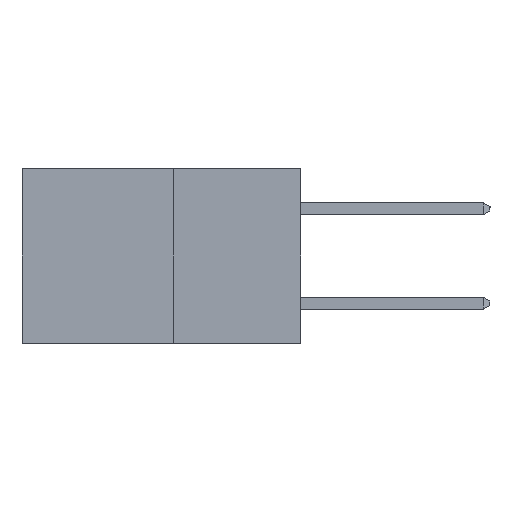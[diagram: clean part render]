
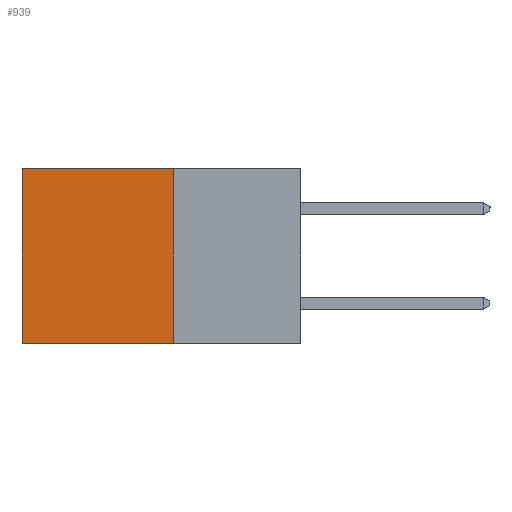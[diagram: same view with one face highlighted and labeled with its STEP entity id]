
A CAD part, left-side view. The second image highlights one B-rep face of the part: STEP entity #939.
In plain terms, the highlighted planar face has unit normal (-1, 0, 0).
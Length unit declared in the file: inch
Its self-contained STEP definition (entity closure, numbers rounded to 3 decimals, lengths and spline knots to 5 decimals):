
#569 = VECTOR ( 'NONE', #7287, 39.37008 ) ;
#777 = CARTESIAN_POINT ( 'NONE',  ( 0.277, 0.27, -0.37 ) ) ;
#939 = ADVANCED_FACE ( 'NONE', ( #9367 ), #11133, .F. ) ;
#1395 = ORIENTED_EDGE ( 'NONE', *, *, #13193, .F. ) ;
#2406 = VERTEX_POINT ( 'NONE', #8641 ) ;
#3998 = VECTOR ( 'NONE', #11134, 39.37008 ) ;
#4005 = VERTEX_POINT ( 'NONE', #13809 ) ;
#4045 = CARTESIAN_POINT ( 'NONE',  ( 0.277, 0.27, -0.37 ) ) ;
#4678 = DIRECTION ( 'NONE',  ( 0., 0., -1. ) ) ;
#5016 = VERTEX_POINT ( 'NONE', #5277 ) ;
#5277 = CARTESIAN_POINT ( 'NONE',  ( 0.277, 0.59, 0. ) ) ;
#5908 = ORIENTED_EDGE ( 'NONE', *, *, #13669, .T. ) ;
#6284 = LINE ( 'NONE', #4045, #6637 ) ;
#6637 = VECTOR ( 'NONE', #13772, 39.37008 ) ;
#7287 = DIRECTION ( 'NONE',  ( 0., 0., -1. ) ) ;
#7516 = AXIS2_PLACEMENT_3D ( 'NONE', #777, #13693, #4678 ) ;
#8641 = CARTESIAN_POINT ( 'NONE',  ( 0.277, 0.27, 0. ) ) ;
#9367 = FACE_OUTER_BOUND ( 'NONE', #10897, .T. ) ;
#9384 = LINE ( 'NONE', #13598, #569 ) ;
#9528 = VECTOR ( 'NONE', #12383, 39.37008 ) ;
#9845 = CARTESIAN_POINT ( 'NONE',  ( 0.277, 0.59, -0.37 ) ) ;
#9855 = LINE ( 'NONE', #11363, #9528 ) ;
#9976 = EDGE_CURVE ( 'NONE', #4005, #11212, #6284, .T. ) ;
#10184 = LINE ( 'NONE', #11086, #3998 ) ;
#10611 = ORIENTED_EDGE ( 'NONE', *, *, #12455, .T. ) ;
#10897 = EDGE_LOOP ( 'NONE', ( #10611, #11290, #1395, #5908 ) ) ;
#11086 = CARTESIAN_POINT ( 'NONE',  ( 0.277, 0.27, 0. ) ) ;
#11133 = PLANE ( 'NONE',  #7516 ) ;
#11134 = DIRECTION ( 'NONE',  ( 0., 1., 0. ) ) ;
#11212 = VERTEX_POINT ( 'NONE', #9845 ) ;
#11290 = ORIENTED_EDGE ( 'NONE', *, *, #9976, .F. ) ;
#11363 = CARTESIAN_POINT ( 'NONE',  ( 0.277, 0.27, -0.37 ) ) ;
#12383 = DIRECTION ( 'NONE',  ( 0., 0., -1. ) ) ;
#12455 = EDGE_CURVE ( 'NONE', #5016, #11212, #9384, .T. ) ;
#13193 = EDGE_CURVE ( 'NONE', #2406, #4005, #9855, .T. ) ;
#13598 = CARTESIAN_POINT ( 'NONE',  ( 0.277, 0.59, -0.37 ) ) ;
#13669 = EDGE_CURVE ( 'NONE', #2406, #5016, #10184, .T. ) ;
#13693 = DIRECTION ( 'NONE',  ( 1., 0., 0. ) ) ;
#13772 = DIRECTION ( 'NONE',  ( 0., 1., 0. ) ) ;
#13809 = CARTESIAN_POINT ( 'NONE',  ( 0.277, 0.27, -0.37 ) ) ;
